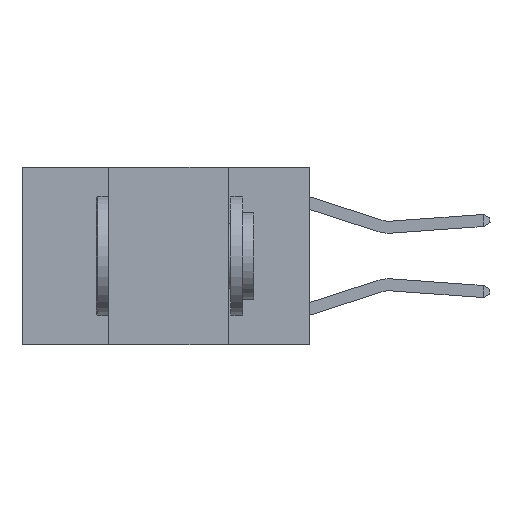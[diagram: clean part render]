
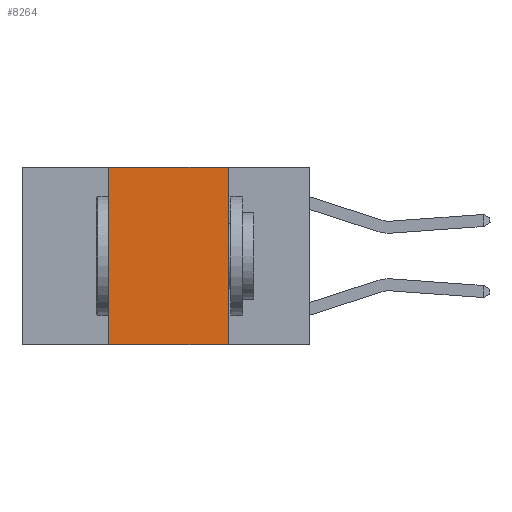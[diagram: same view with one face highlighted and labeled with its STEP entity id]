
A CAD part, left-side view. The second image highlights one B-rep face of the part: STEP entity #8264.
In plain terms, the highlighted planar face has unit normal (-1, 0, 0).
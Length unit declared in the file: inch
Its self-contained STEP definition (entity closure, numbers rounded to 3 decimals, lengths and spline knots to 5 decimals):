
#1102 = FACE_OUTER_BOUND ( 'NONE', #8493, .T. ) ;
#2197 = CARTESIAN_POINT ( 'NONE',  ( 0., 0.42, 0. ) ) ;
#2924 = CARTESIAN_POINT ( 'NONE',  ( 0., 0.17, 0. ) ) ;
#3867 = CARTESIAN_POINT ( 'NONE',  ( 0., 0.17, 0. ) ) ;
#4124 = DIRECTION ( 'NONE',  ( 0., 0., 1. ) ) ;
#5135 = ORIENTED_EDGE ( 'NONE', *, *, #30367, .F. ) ;
#8236 = CARTESIAN_POINT ( 'NONE',  ( 0., 0.42, -0.37 ) ) ;
#8264 = ADVANCED_FACE ( 'NONE', ( #1102 ), #12829, .F. ) ;
#8410 = VECTOR ( 'NONE', #26536, 39.37008 ) ;
#8493 = EDGE_LOOP ( 'NONE', ( #13494, #5135, #13049, #24681 ) ) ;
#9820 = LINE ( 'NONE', #12321, #28046 ) ;
#11822 = EDGE_CURVE ( 'NONE', #17043, #27974, #23006, .T. ) ;
#12321 = CARTESIAN_POINT ( 'NONE',  ( 0., 0.6, -0.37 ) ) ;
#12829 = PLANE ( 'NONE',  #27332 ) ;
#13043 = EDGE_CURVE ( 'NONE', #17043, #20941, #9820, .T. ) ;
#13048 = VERTEX_POINT ( 'NONE', #2924 ) ;
#13049 = ORIENTED_EDGE ( 'NONE', *, *, #11822, .F. ) ;
#13494 = ORIENTED_EDGE ( 'NONE', *, *, #29764, .F. ) ;
#14567 = CARTESIAN_POINT ( 'NONE',  ( 0., 0.6, 0. ) ) ;
#15087 = VECTOR ( 'NONE', #4124, 39.37008 ) ;
#15337 = CARTESIAN_POINT ( 'NONE',  ( 0., 0.6, 0. ) ) ;
#15797 = DIRECTION ( 'NONE',  ( 0., 0., -1. ) ) ;
#16223 = LINE ( 'NONE', #3867, #23348 ) ;
#17043 = VERTEX_POINT ( 'NONE', #8236 ) ;
#17054 = LINE ( 'NONE', #14567, #8410 ) ;
#17460 = DIRECTION ( 'NONE',  ( 0., -1., 0. ) ) ;
#20101 = CARTESIAN_POINT ( 'NONE',  ( 0., 0.17, -0.37 ) ) ;
#20941 = VERTEX_POINT ( 'NONE', #20101 ) ;
#23006 = LINE ( 'NONE', #25190, #15087 ) ;
#23348 = VECTOR ( 'NONE', #30092, 39.37008 ) ;
#24681 = ORIENTED_EDGE ( 'NONE', *, *, #13043, .T. ) ;
#25190 = CARTESIAN_POINT ( 'NONE',  ( 0., 0.42, 0. ) ) ;
#26536 = DIRECTION ( 'NONE',  ( 0., -1., 0. ) ) ;
#27332 = AXIS2_PLACEMENT_3D ( 'NONE', #15337, #29815, #15797 ) ;
#27974 = VERTEX_POINT ( 'NONE', #2197 ) ;
#28046 = VECTOR ( 'NONE', #17460, 39.37008 ) ;
#29764 = EDGE_CURVE ( 'NONE', #13048, #20941, #16223, .T. ) ;
#29815 = DIRECTION ( 'NONE',  ( 1., 0., 0. ) ) ;
#30092 = DIRECTION ( 'NONE',  ( 0., 0., -1. ) ) ;
#30367 = EDGE_CURVE ( 'NONE', #27974, #13048, #17054, .T. ) ;
